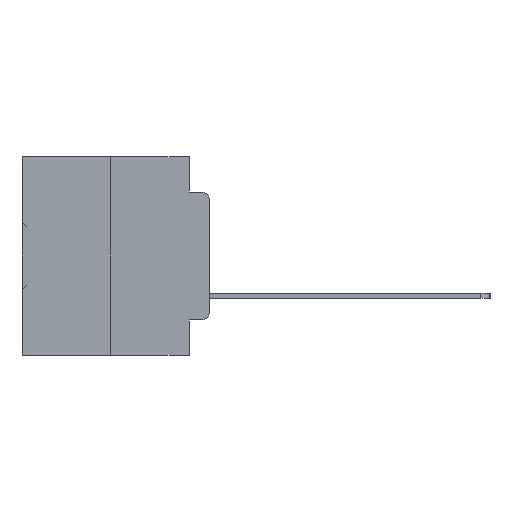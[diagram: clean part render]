
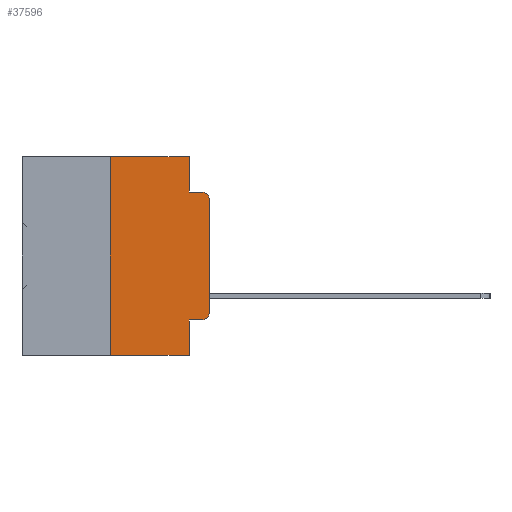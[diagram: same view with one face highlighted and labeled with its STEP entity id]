
A CAD part, left-side view. The second image highlights one B-rep face of the part: STEP entity #37596.
In plain terms, the highlighted planar face has unit normal (-1, 0, 0).
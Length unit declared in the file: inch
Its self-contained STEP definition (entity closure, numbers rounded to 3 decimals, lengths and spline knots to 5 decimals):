
#261 = VERTEX_POINT ( 'NONE', #21731 ) ;
#315 = EDGE_LOOP ( 'NONE', ( #29738, #1714, #3144, #14824, #800, #17170, #12034, #7890, #32636, #26535 ) ) ;
#683 = CIRCLE ( 'NONE', #18614, 0.02 ) ;
#774 = CARTESIAN_POINT ( 'NONE',  ( 0., 0.02, -0.4115 ) ) ;
#800 = ORIENTED_EDGE ( 'NONE', *, *, #10934, .F. ) ;
#1022 = EDGE_CURVE ( 'NONE', #261, #21620, #16204, .T. ) ;
#1714 = ORIENTED_EDGE ( 'NONE', *, *, #21066, .T. ) ;
#1803 = DIRECTION ( 'NONE',  ( 0., 0., -1. ) ) ;
#2738 = AXIS2_PLACEMENT_3D ( 'NONE', #9945, #27945, #10079 ) ;
#3144 = ORIENTED_EDGE ( 'NONE', *, *, #19049, .F. ) ;
#3410 = LINE ( 'NONE', #19510, #9482 ) ;
#3677 = DIRECTION ( 'NONE',  ( 0., -1., 0. ) ) ;
#4475 = VECTOR ( 'NONE', #3677, 39.37008 ) ;
#5528 = DIRECTION ( 'NONE',  ( 0., 0., 1. ) ) ;
#5905 = EDGE_CURVE ( 'NONE', #261, #20440, #11652, .T. ) ;
#6019 = LINE ( 'NONE', #20324, #11999 ) ;
#6072 = LINE ( 'NONE', #28948, #20917 ) ;
#6094 = VERTEX_POINT ( 'NONE', #18008 ) ;
#6124 = VERTEX_POINT ( 'NONE', #12154 ) ;
#7146 = EDGE_CURVE ( 'NONE', #6094, #35453, #6072, .T. ) ;
#7399 = CARTESIAN_POINT ( 'NONE',  ( 0., 0.051, -0.4115 ) ) ;
#7890 = ORIENTED_EDGE ( 'NONE', *, *, #5905, .F. ) ;
#8684 = DIRECTION ( 'NONE',  ( 0., -1., 0. ) ) ;
#9148 = VERTEX_POINT ( 'NONE', #30776 ) ;
#9482 = VECTOR ( 'NONE', #28419, 39.37008 ) ;
#9873 = DIRECTION ( 'NONE',  ( -1., 0., 0. ) ) ;
#9945 = CARTESIAN_POINT ( 'NONE',  ( 0., 0.473, 0. ) ) ;
#10079 = DIRECTION ( 'NONE',  ( 0., 0., -1. ) ) ;
#10739 = CARTESIAN_POINT ( 'NONE',  ( 0., 0.051, -0.5 ) ) ;
#10934 = EDGE_CURVE ( 'NONE', #18389, #6094, #15080, .T. ) ;
#11652 = LINE ( 'NONE', #17131, #19564 ) ;
#11999 = VECTOR ( 'NONE', #5528, 39.37008 ) ;
#12034 = ORIENTED_EDGE ( 'NONE', *, *, #25837, .T. ) ;
#12154 = CARTESIAN_POINT ( 'NONE',  ( 0., 0.02, -0.0885 ) ) ;
#12937 = PLANE ( 'NONE',  #2738 ) ;
#13190 = CARTESIAN_POINT ( 'NONE',  ( 0., 0.25, 0. ) ) ;
#14173 = VECTOR ( 'NONE', #8684, 39.37008 ) ;
#14538 = CARTESIAN_POINT ( 'NONE',  ( 0., 0.473, 0. ) ) ;
#14824 = ORIENTED_EDGE ( 'NONE', *, *, #7146, .F. ) ;
#15080 = LINE ( 'NONE', #14538, #14173 ) ;
#15508 = CARTESIAN_POINT ( 'NONE',  ( 0., 0.051, -0.0885 ) ) ;
#16204 = LINE ( 'NONE', #7399, #23214 ) ;
#17131 = CARTESIAN_POINT ( 'NONE',  ( 0., 0.051, 0. ) ) ;
#17170 = ORIENTED_EDGE ( 'NONE', *, *, #23817, .F. ) ;
#17414 = CARTESIAN_POINT ( 'NONE',  ( 0., 0., -0.3915 ) ) ;
#18008 = CARTESIAN_POINT ( 'NONE',  ( 0., 0.051, 0. ) ) ;
#18389 = VERTEX_POINT ( 'NONE', #13190 ) ;
#18614 = AXIS2_PLACEMENT_3D ( 'NONE', #37507, #19644, #1803 ) ;
#19049 = EDGE_CURVE ( 'NONE', #35453, #6124, #36157, .T. ) ;
#19282 = VECTOR ( 'NONE', #27910, 39.37008 ) ;
#19510 = CARTESIAN_POINT ( 'NONE',  ( 0., 0., 0. ) ) ;
#19564 = VECTOR ( 'NONE', #20123, 39.37008 ) ;
#19644 = DIRECTION ( 'NONE',  ( -1., 0., 0. ) ) ;
#19748 = EDGE_CURVE ( 'NONE', #21620, #28524, #28678, .T. ) ;
#20123 = DIRECTION ( 'NONE',  ( 0., 0., -1. ) ) ;
#20324 = CARTESIAN_POINT ( 'NONE',  ( 0., 0.25, 0. ) ) ;
#20440 = VERTEX_POINT ( 'NONE', #10739 ) ;
#20917 = VECTOR ( 'NONE', #23031, 39.37008 ) ;
#21066 = EDGE_CURVE ( 'NONE', #33136, #6124, #683, .T. ) ;
#21588 = AXIS2_PLACEMENT_3D ( 'NONE', #27730, #9873, #30768 ) ;
#21620 = VERTEX_POINT ( 'NONE', #774 ) ;
#21731 = CARTESIAN_POINT ( 'NONE',  ( 0., 0.051, -0.4115 ) ) ;
#22329 = EDGE_CURVE ( 'NONE', #28524, #33136, #3410, .T. ) ;
#23031 = DIRECTION ( 'NONE',  ( 0., 0., -1. ) ) ;
#23214 = VECTOR ( 'NONE', #34251, 39.37008 ) ;
#23817 = EDGE_CURVE ( 'NONE', #9148, #18389, #6019, .T. ) ;
#24308 = CARTESIAN_POINT ( 'NONE',  ( 0., 0., -0.1085 ) ) ;
#24875 = CARTESIAN_POINT ( 'NONE',  ( 0., 0.473, -0.5 ) ) ;
#25837 = EDGE_CURVE ( 'NONE', #9148, #20440, #28201, .T. ) ;
#26535 = ORIENTED_EDGE ( 'NONE', *, *, #19748, .T. ) ;
#27730 = CARTESIAN_POINT ( 'NONE',  ( 0., 0.02, -0.3915 ) ) ;
#27910 = DIRECTION ( 'NONE',  ( 0., -1., 0. ) ) ;
#27945 = DIRECTION ( 'NONE',  ( 1., 0., 0. ) ) ;
#28201 = LINE ( 'NONE', #24875, #19282 ) ;
#28419 = DIRECTION ( 'NONE',  ( 0., 0., 1. ) ) ;
#28524 = VERTEX_POINT ( 'NONE', #17414 ) ;
#28678 = CIRCLE ( 'NONE', #21588, 0.02 ) ;
#28948 = CARTESIAN_POINT ( 'NONE',  ( 0., 0.051, 0. ) ) ;
#29738 = ORIENTED_EDGE ( 'NONE', *, *, #22329, .T. ) ;
#30768 = DIRECTION ( 'NONE',  ( 0., 0., -1. ) ) ;
#30776 = CARTESIAN_POINT ( 'NONE',  ( 0., 0.25, -0.5 ) ) ;
#32636 = ORIENTED_EDGE ( 'NONE', *, *, #1022, .T. ) ;
#33136 = VERTEX_POINT ( 'NONE', #24308 ) ;
#34251 = DIRECTION ( 'NONE',  ( 0., -1., 0. ) ) ;
#35453 = VERTEX_POINT ( 'NONE', #38329 ) ;
#36052 = FACE_OUTER_BOUND ( 'NONE', #315, .T. ) ;
#36157 = LINE ( 'NONE', #15508, #4475 ) ;
#37507 = CARTESIAN_POINT ( 'NONE',  ( 0., 0.02, -0.1085 ) ) ;
#37596 = ADVANCED_FACE ( 'NONE', ( #36052 ), #12937, .F. ) ;
#38329 = CARTESIAN_POINT ( 'NONE',  ( 0., 0.051, -0.0885 ) ) ;
